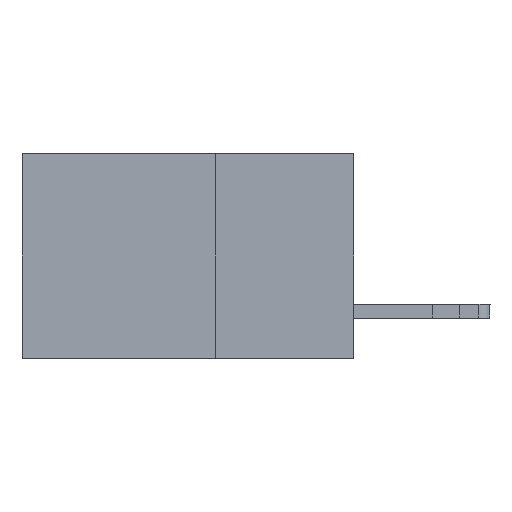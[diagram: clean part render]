
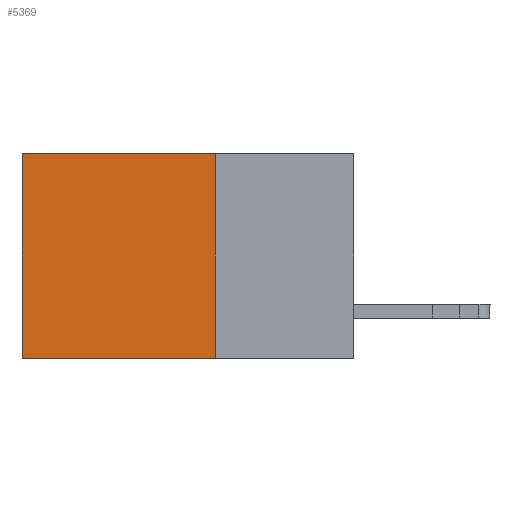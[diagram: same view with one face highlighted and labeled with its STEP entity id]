
A CAD part, left-side view. The second image highlights one B-rep face of the part: STEP entity #5369.
In plain terms, the highlighted planar face has unit normal (-1, 0, 0).
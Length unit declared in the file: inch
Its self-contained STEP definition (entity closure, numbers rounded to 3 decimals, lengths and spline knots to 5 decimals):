
#572 = DIRECTION ( 'NONE',  ( 0., 1., 0. ) ) ;
#1053 = VERTEX_POINT ( 'NONE', #4940 ) ;
#1594 = EDGE_CURVE ( 'NONE', #2950, #1053, #14965, .T. ) ;
#1696 = EDGE_LOOP ( 'NONE', ( #6150, #13590, #4840, #7969 ) ) ;
#2016 = CARTESIAN_POINT ( 'NONE',  ( 0.2875, 0.25, -0.37 ) ) ;
#2172 = DIRECTION ( 'NONE',  ( 0., 0., -1. ) ) ;
#2307 = FACE_OUTER_BOUND ( 'NONE', #1696, .T. ) ;
#2482 = DIRECTION ( 'NONE',  ( 0., 0., -1. ) ) ;
#2670 = CARTESIAN_POINT ( 'NONE',  ( 0.2875, 0.25, -0.37 ) ) ;
#2678 = LINE ( 'NONE', #8460, #10951 ) ;
#2947 = VERTEX_POINT ( 'NONE', #4107 ) ;
#2950 = VERTEX_POINT ( 'NONE', #2670 ) ;
#3894 = CARTESIAN_POINT ( 'NONE',  ( 0.2875, 0.25, 0. ) ) ;
#4107 = CARTESIAN_POINT ( 'NONE',  ( 0.2875, 0.6, 0. ) ) ;
#4278 = CARTESIAN_POINT ( 'NONE',  ( 0.2875, 0.25, 0. ) ) ;
#4840 = ORIENTED_EDGE ( 'NONE', *, *, #14447, .F. ) ;
#4940 = CARTESIAN_POINT ( 'NONE',  ( 0.2875, 0.6, -0.37 ) ) ;
#5082 = CARTESIAN_POINT ( 'NONE',  ( 0.2875, 0.25, 0. ) ) ;
#5369 = ADVANCED_FACE ( 'NONE', ( #2307 ), #12455, .F. ) ;
#6150 = ORIENTED_EDGE ( 'NONE', *, *, #15212, .T. ) ;
#6307 = VECTOR ( 'NONE', #2172, 39.37008 ) ;
#6998 = LINE ( 'NONE', #5082, #6307 ) ;
#7533 = AXIS2_PLACEMENT_3D ( 'NONE', #3894, #9642, #16515 ) ;
#7969 = ORIENTED_EDGE ( 'NONE', *, *, #18123, .T. ) ;
#8095 = VECTOR ( 'NONE', #572, 39.37008 ) ;
#8460 = CARTESIAN_POINT ( 'NONE',  ( 0.2875, 0.6, 0. ) ) ;
#9642 = DIRECTION ( 'NONE',  ( 1., 0., 0. ) ) ;
#10076 = DIRECTION ( 'NONE',  ( 0., 1., 0. ) ) ;
#10951 = VECTOR ( 'NONE', #2482, 39.37008 ) ;
#12251 = VERTEX_POINT ( 'NONE', #15732 ) ;
#12455 = PLANE ( 'NONE',  #7533 ) ;
#13590 = ORIENTED_EDGE ( 'NONE', *, *, #1594, .F. ) ;
#14418 = VECTOR ( 'NONE', #10076, 39.37008 ) ;
#14447 = EDGE_CURVE ( 'NONE', #12251, #2950, #6998, .T. ) ;
#14965 = LINE ( 'NONE', #2016, #8095 ) ;
#15212 = EDGE_CURVE ( 'NONE', #2947, #1053, #2678, .T. ) ;
#15732 = CARTESIAN_POINT ( 'NONE',  ( 0.2875, 0.25, 0. ) ) ;
#16515 = DIRECTION ( 'NONE',  ( 0., 0., -1. ) ) ;
#18123 = EDGE_CURVE ( 'NONE', #12251, #2947, #18209, .T. ) ;
#18209 = LINE ( 'NONE', #4278, #14418 ) ;
